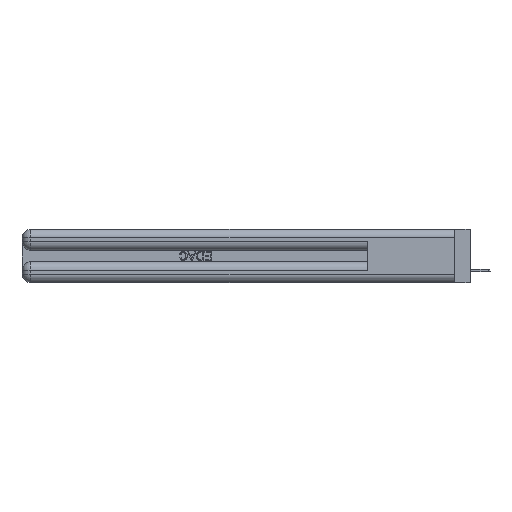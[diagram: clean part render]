
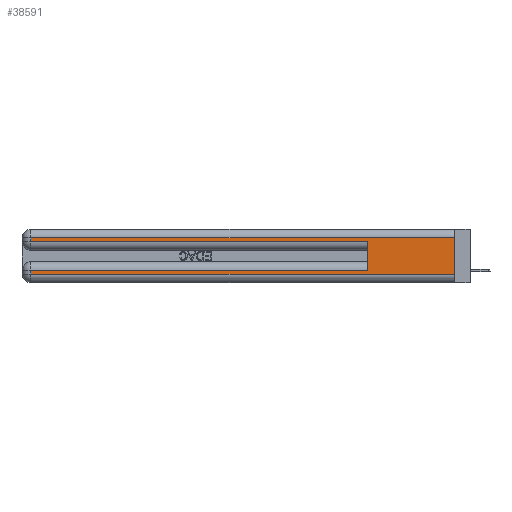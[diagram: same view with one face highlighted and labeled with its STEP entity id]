
A CAD part, left-side view. The second image highlights one B-rep face of the part: STEP entity #38591.
In plain terms, the highlighted planar face has unit normal (-1, 0, 0).
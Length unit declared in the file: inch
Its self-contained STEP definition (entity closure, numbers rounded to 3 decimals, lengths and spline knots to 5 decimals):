
#470 = CARTESIAN_POINT ( 'NONE',  ( 0., 0., 0.06 ) ) ;
#681 = LINE ( 'NONE', #24177, #19477 ) ;
#946 = DIRECTION ( 'NONE',  ( 1., 0., 0. ) ) ;
#1175 = VERTEX_POINT ( 'NONE', #35288 ) ;
#1201 = CARTESIAN_POINT ( 'NONE',  ( 0., 0., 0.37 ) ) ;
#1675 = ORIENTED_EDGE ( 'NONE', *, *, #3413, .T. ) ;
#1947 = LINE ( 'NONE', #2700, #8941 ) ;
#2700 = CARTESIAN_POINT ( 'NONE',  ( 0., 2.94, 0.37 ) ) ;
#3413 = EDGE_CURVE ( 'NONE', #22984, #42426, #1947, .T. ) ;
#5491 = FACE_OUTER_BOUND ( 'NONE', #9408, .T. ) ;
#6328 = CARTESIAN_POINT ( 'NONE',  ( 0., 0., 0.06 ) ) ;
#7001 = VECTOR ( 'NONE', #21728, 39.37008 ) ;
#7038 = LINE ( 'NONE', #11306, #41530 ) ;
#7959 = VERTEX_POINT ( 'NONE', #26407 ) ;
#8093 = ORIENTED_EDGE ( 'NONE', *, *, #25392, .T. ) ;
#8415 = VERTEX_POINT ( 'NONE', #38645 ) ;
#8941 = VECTOR ( 'NONE', #41120, 39.37008 ) ;
#8998 = EDGE_CURVE ( 'NONE', #8415, #12590, #681, .T. ) ;
#9408 = EDGE_LOOP ( 'NONE', ( #44294, #37281, #1675, #43846, #27737, #23660, #29071, #8093 ) ) ;
#10164 = EDGE_CURVE ( 'NONE', #42426, #28501, #7038, .T. ) ;
#10441 = EDGE_CURVE ( 'NONE', #7959, #1175, #10962, .T. ) ;
#10962 = LINE ( 'NONE', #22349, #46369 ) ;
#11306 = CARTESIAN_POINT ( 'NONE',  ( 0., 0., 0.285 ) ) ;
#12590 = VERTEX_POINT ( 'NONE', #470 ) ;
#14193 = VERTEX_POINT ( 'NONE', #27447 ) ;
#15707 = EDGE_CURVE ( 'NONE', #14193, #28501, #32224, .T. ) ;
#18537 = DIRECTION ( 'NONE',  ( 0., 0., -1. ) ) ;
#19477 = VECTOR ( 'NONE', #39846, 39.37008 ) ;
#20369 = CARTESIAN_POINT ( 'NONE',  ( 0., 0.6, 0.145 ) ) ;
#20986 = DIRECTION ( 'NONE',  ( 0., 1., 0. ) ) ;
#21728 = DIRECTION ( 'NONE',  ( 0., -1., 0. ) ) ;
#22349 = CARTESIAN_POINT ( 'NONE',  ( 0., 2.94, 0.37 ) ) ;
#22868 = DIRECTION ( 'NONE',  ( 0., 1., 0. ) ) ;
#22984 = VERTEX_POINT ( 'NONE', #40561 ) ;
#23660 = ORIENTED_EDGE ( 'NONE', *, *, #49676, .T. ) ;
#24177 = CARTESIAN_POINT ( 'NONE',  ( 0., 0., 0.37 ) ) ;
#24814 = AXIS2_PLACEMENT_3D ( 'NONE', #1201, #946, #43914 ) ;
#25235 = EDGE_CURVE ( 'NONE', #8415, #22984, #27799, .T. ) ;
#25392 = EDGE_CURVE ( 'NONE', #1175, #12590, #40953, .T. ) ;
#26407 = CARTESIAN_POINT ( 'NONE',  ( 0., 2.94, 0.085 ) ) ;
#26496 = CARTESIAN_POINT ( 'NONE',  ( 0., 0.6, 0.285 ) ) ;
#27223 = DIRECTION ( 'NONE',  ( 0., -1., 0. ) ) ;
#27447 = CARTESIAN_POINT ( 'NONE',  ( 0., 0.6, 0.085 ) ) ;
#27737 = ORIENTED_EDGE ( 'NONE', *, *, #15707, .F. ) ;
#27799 = LINE ( 'NONE', #47044, #37606 ) ;
#28321 = VECTOR ( 'NONE', #43385, 39.37008 ) ;
#28484 = PLANE ( 'NONE',  #24814 ) ;
#28501 = VERTEX_POINT ( 'NONE', #26496 ) ;
#29071 = ORIENTED_EDGE ( 'NONE', *, *, #10441, .T. ) ;
#30055 = VECTOR ( 'NONE', #22868, 39.37008 ) ;
#31194 = LINE ( 'NONE', #42855, #30055 ) ;
#32224 = LINE ( 'NONE', #20369, #28321 ) ;
#35288 = CARTESIAN_POINT ( 'NONE',  ( 0., 2.94, 0.06 ) ) ;
#37281 = ORIENTED_EDGE ( 'NONE', *, *, #25235, .T. ) ;
#37606 = VECTOR ( 'NONE', #20986, 39.37008 ) ;
#38591 = ADVANCED_FACE ( 'NONE', ( #5491 ), #28484, .F. ) ;
#38645 = CARTESIAN_POINT ( 'NONE',  ( 0., 0., 0.31 ) ) ;
#39846 = DIRECTION ( 'NONE',  ( 0., 0., -1. ) ) ;
#40561 = CARTESIAN_POINT ( 'NONE',  ( 0., 2.94, 0.31 ) ) ;
#40953 = LINE ( 'NONE', #6328, #7001 ) ;
#41120 = DIRECTION ( 'NONE',  ( 0., 0., -1. ) ) ;
#41530 = VECTOR ( 'NONE', #27223, 39.37008 ) ;
#42426 = VERTEX_POINT ( 'NONE', #46477 ) ;
#42855 = CARTESIAN_POINT ( 'NONE',  ( 0., 0., 0.085 ) ) ;
#43385 = DIRECTION ( 'NONE',  ( 0., 0., 1. ) ) ;
#43846 = ORIENTED_EDGE ( 'NONE', *, *, #10164, .T. ) ;
#43914 = DIRECTION ( 'NONE',  ( 0., 0., -1. ) ) ;
#44294 = ORIENTED_EDGE ( 'NONE', *, *, #8998, .F. ) ;
#46369 = VECTOR ( 'NONE', #18537, 39.37008 ) ;
#46477 = CARTESIAN_POINT ( 'NONE',  ( 0., 2.94, 0.285 ) ) ;
#47044 = CARTESIAN_POINT ( 'NONE',  ( 0., 0., 0.31 ) ) ;
#49676 = EDGE_CURVE ( 'NONE', #14193, #7959, #31194, .T. ) ;
